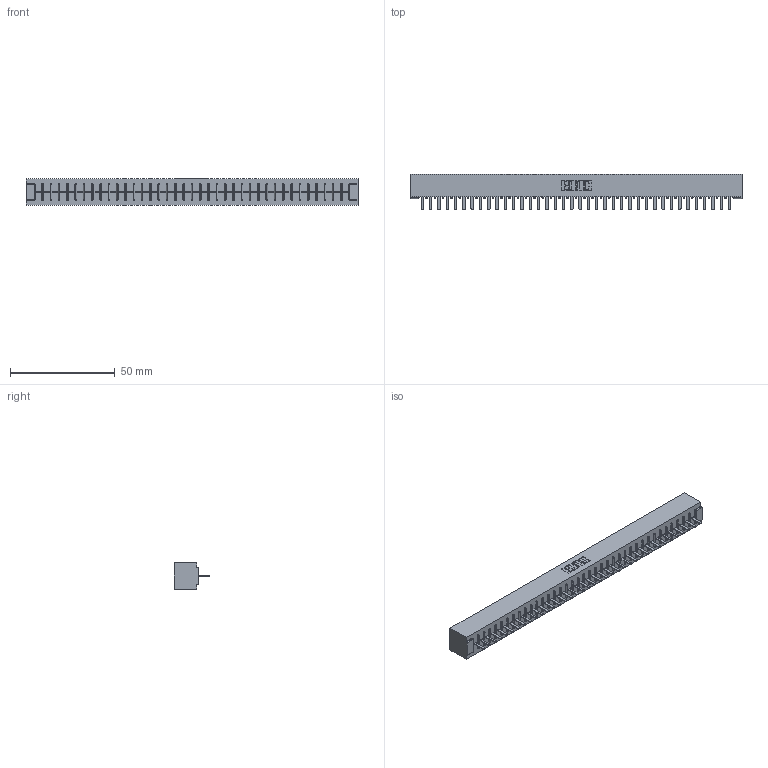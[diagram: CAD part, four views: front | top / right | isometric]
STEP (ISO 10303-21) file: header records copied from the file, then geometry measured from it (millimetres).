
FILE_DESCRIPTION (( 'STEP AP203' ), '1' );
FILE_NAME ('316-038-420-101.STEP', '2020-09-23T05:48:36', ( '' ), ( '' ), 'SwSTEP 2.0', 'SolidWorks 2020', '' );
FILE_SCHEMA (( 'CONFIG_CONTROL_DESIGN' ));
Length unit declared in the file: inch
Products named in the file (3): 306-290-001_120; 306 Part_No Mounting; 316-038-420-101
Assembly tree (39 placements, depth 2):
  316-038-420-101
    306 Part_No Mounting
    306-290-001_120  x38
Bounding box: 158.45 x 17.12 x 12.7 mm (x, y, z)
Volume: 18078.1 mm3; surface area: 18657.3 mm2
Topology: 39 solids, 39 shells, 2768 faces, 7778 edges, 4980 vertices
Faces by surface type: plane 1850, cylinder 766, sphere 152
Entity records: 35633 total; most frequent: CARTESIAN_POINT 5981, ORIENTED_EDGE 5928, DIRECTION 5898, EDGE_CURVE 2964, LINE 2320, VECTOR 2320, VERTEX_POINT 1872, AXIS2_PLACEMENT_3D 1789
